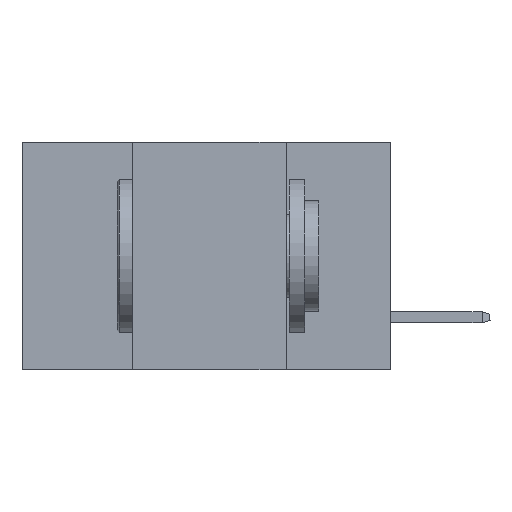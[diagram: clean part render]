
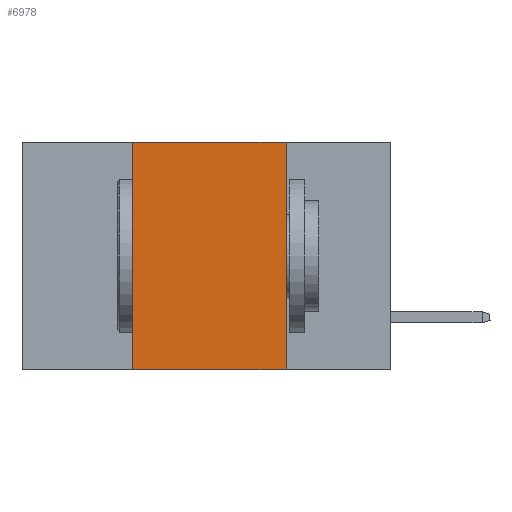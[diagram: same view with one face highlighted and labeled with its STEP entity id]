
A CAD part, left-side view. The second image highlights one B-rep face of the part: STEP entity #6978.
In plain terms, the highlighted planar face has unit normal (-1, 0, 0).
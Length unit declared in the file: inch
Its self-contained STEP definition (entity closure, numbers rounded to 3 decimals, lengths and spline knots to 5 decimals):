
#34 = DIRECTION ( 'NONE',  ( 0., 0., -1. ) ) ;
#274 = CARTESIAN_POINT ( 'NONE',  ( 0., 0.17, 0. ) ) ;
#355 = FACE_OUTER_BOUND ( 'NONE', #10904, .T. ) ;
#358 = LINE ( 'NONE', #274, #6757 ) ;
#1060 = DIRECTION ( 'NONE',  ( 0., 0., 1. ) ) ;
#1199 = LINE ( 'NONE', #6753, #8278 ) ;
#2058 = CARTESIAN_POINT ( 'NONE',  ( 0., 0.17, -0.37 ) ) ;
#2374 = VERTEX_POINT ( 'NONE', #4759 ) ;
#2409 = VERTEX_POINT ( 'NONE', #2058 ) ;
#2905 = LINE ( 'NONE', #11409, #9858 ) ;
#3085 = AXIS2_PLACEMENT_3D ( 'NONE', #4123, #5322, #34 ) ;
#3189 = VERTEX_POINT ( 'NONE', #9662 ) ;
#3312 = DIRECTION ( 'NONE',  ( 0., -1., 0. ) ) ;
#3328 = VECTOR ( 'NONE', #7740, 39.37008 ) ;
#3426 = ORIENTED_EDGE ( 'NONE', *, *, #8040, .F. ) ;
#3808 = DIRECTION ( 'NONE',  ( 0., 0., -1. ) ) ;
#4123 = CARTESIAN_POINT ( 'NONE',  ( 0., 0.6, 0. ) ) ;
#4181 = ORIENTED_EDGE ( 'NONE', *, *, #5089, .F. ) ;
#4312 = VERTEX_POINT ( 'NONE', #4522 ) ;
#4522 = CARTESIAN_POINT ( 'NONE',  ( 0., 0.42, 0. ) ) ;
#4759 = CARTESIAN_POINT ( 'NONE',  ( 0., 0.42, -0.37 ) ) ;
#5089 = EDGE_CURVE ( 'NONE', #4312, #3189, #2905, .T. ) ;
#5322 = DIRECTION ( 'NONE',  ( 1., 0., 0. ) ) ;
#6753 = CARTESIAN_POINT ( 'NONE',  ( 0., 0.42, 0. ) ) ;
#6757 = VECTOR ( 'NONE', #3808, 39.37008 ) ;
#6978 = ADVANCED_FACE ( 'NONE', ( #355 ), #9555, .F. ) ;
#7522 = LINE ( 'NONE', #11299, #3328 ) ;
#7598 = EDGE_CURVE ( 'NONE', #3189, #2409, #358, .T. ) ;
#7740 = DIRECTION ( 'NONE',  ( 0., -1., 0. ) ) ;
#8040 = EDGE_CURVE ( 'NONE', #2374, #4312, #1199, .T. ) ;
#8168 = ORIENTED_EDGE ( 'NONE', *, *, #10871, .T. ) ;
#8278 = VECTOR ( 'NONE', #1060, 39.37008 ) ;
#9555 = PLANE ( 'NONE',  #3085 ) ;
#9662 = CARTESIAN_POINT ( 'NONE',  ( 0., 0.17, 0. ) ) ;
#9709 = ORIENTED_EDGE ( 'NONE', *, *, #7598, .F. ) ;
#9858 = VECTOR ( 'NONE', #3312, 39.37008 ) ;
#10871 = EDGE_CURVE ( 'NONE', #2374, #2409, #7522, .T. ) ;
#10904 = EDGE_LOOP ( 'NONE', ( #9709, #4181, #3426, #8168 ) ) ;
#11299 = CARTESIAN_POINT ( 'NONE',  ( 0., 0.6, -0.37 ) ) ;
#11409 = CARTESIAN_POINT ( 'NONE',  ( 0., 0.6, 0. ) ) ;
